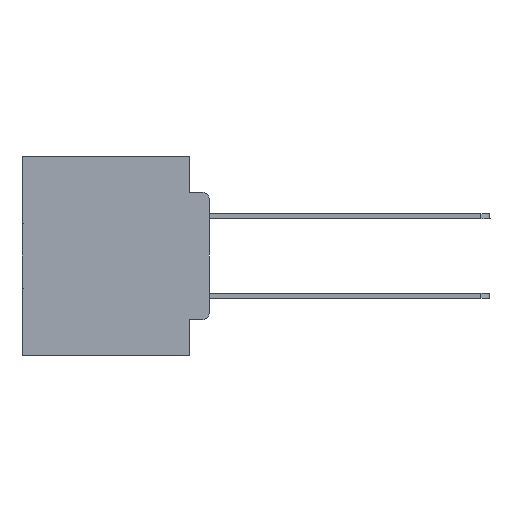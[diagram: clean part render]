
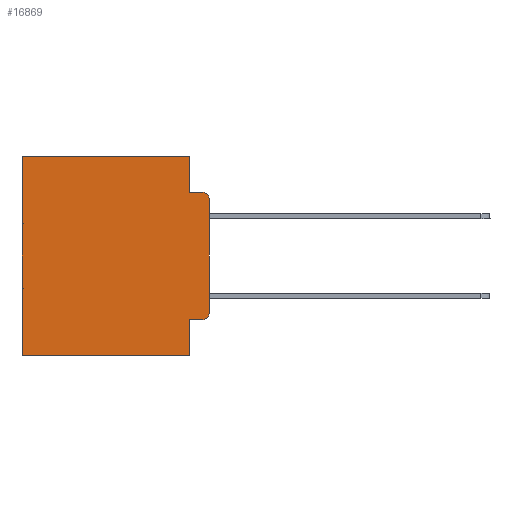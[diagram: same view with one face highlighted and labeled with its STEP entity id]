
A CAD part, left-side view. The second image highlights one B-rep face of the part: STEP entity #16869.
In plain terms, the highlighted planar face has unit normal (-1, 0, 0).
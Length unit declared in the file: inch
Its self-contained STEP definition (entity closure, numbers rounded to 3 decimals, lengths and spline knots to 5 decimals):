
#1502 = VERTEX_POINT ( 'NONE', #21563 ) ;
#1504 = VERTEX_POINT ( 'NONE', #26779 ) ;
#1955 = LINE ( 'NONE', #20442, #27430 ) ;
#2337 = EDGE_CURVE ( 'NONE', #17889, #27741, #2546, .T. ) ;
#2368 = DIRECTION ( 'NONE',  ( 1., 0., 0. ) ) ;
#2546 = LINE ( 'NONE', #7287, #12691 ) ;
#4616 = VERTEX_POINT ( 'NONE', #29684 ) ;
#5241 = VECTOR ( 'NONE', #23494, 39.37008 ) ;
#5605 = VECTOR ( 'NONE', #20570, 39.37008 ) ;
#6150 = AXIS2_PLACEMENT_3D ( 'NONE', #28214, #13589, #30662 ) ;
#6240 = CARTESIAN_POINT ( 'NONE',  ( 0.298, 0., 0. ) ) ;
#6424 = VERTEX_POINT ( 'NONE', #9900 ) ;
#6733 = CARTESIAN_POINT ( 'NONE',  ( 0.298, 0.473, 0. ) ) ;
#7261 = CARTESIAN_POINT ( 'NONE',  ( 0.298, 0., 0. ) ) ;
#7287 = CARTESIAN_POINT ( 'NONE',  ( 0.298, 0.051, -0.0885 ) ) ;
#7457 = DIRECTION ( 'NONE',  ( 0., -1., 0. ) ) ;
#7650 = LINE ( 'NONE', #17932, #9225 ) ;
#8582 = ORIENTED_EDGE ( 'NONE', *, *, #15921, .T. ) ;
#8660 = EDGE_CURVE ( 'NONE', #6424, #27741, #17504, .T. ) ;
#8824 = CARTESIAN_POINT ( 'NONE',  ( 0.298, 0.02, -0.3915 ) ) ;
#8850 = CARTESIAN_POINT ( 'NONE',  ( 0.298, 0.051, 0. ) ) ;
#9006 = EDGE_CURVE ( 'NONE', #14429, #17889, #31174, .T. ) ;
#9225 = VECTOR ( 'NONE', #25160, 39.37008 ) ;
#9534 = CARTESIAN_POINT ( 'NONE',  ( 0.298, 0., -0.5 ) ) ;
#9900 = CARTESIAN_POINT ( 'NONE',  ( 0.298, 0., -0.1085 ) ) ;
#10178 = ORIENTED_EDGE ( 'NONE', *, *, #29136, .T. ) ;
#10765 = DIRECTION ( 'NONE',  ( 0., 0., -1. ) ) ;
#11362 = DIRECTION ( 'NONE',  ( 0., 0., -1. ) ) ;
#11658 = VECTOR ( 'NONE', #10765, 39.37008 ) ;
#11864 = LINE ( 'NONE', #6240, #5241 ) ;
#12130 = DIRECTION ( 'NONE',  ( 0., -1., 0. ) ) ;
#12381 = CARTESIAN_POINT ( 'NONE',  ( 0.298, 0.473, -0.5 ) ) ;
#12691 = VECTOR ( 'NONE', #7457, 39.37008 ) ;
#12758 = EDGE_LOOP ( 'NONE', ( #29156, #12996, #13182, #12908, #10178, #31311, #23656, #28726, #15847, #8582 ) ) ;
#12908 = ORIENTED_EDGE ( 'NONE', *, *, #9006, .F. ) ;
#12996 = ORIENTED_EDGE ( 'NONE', *, *, #8660, .T. ) ;
#13182 = ORIENTED_EDGE ( 'NONE', *, *, #2337, .F. ) ;
#13232 = CIRCLE ( 'NONE', #23271, 0.02 ) ;
#13515 = LINE ( 'NONE', #26816, #20838 ) ;
#13589 = DIRECTION ( 'NONE',  ( -1., 0., 0. ) ) ;
#14429 = VERTEX_POINT ( 'NONE', #8850 ) ;
#15496 = EDGE_CURVE ( 'NONE', #21499, #31439, #24745, .T. ) ;
#15612 = DIRECTION ( 'NONE',  ( 0., 0., -1. ) ) ;
#15847 = ORIENTED_EDGE ( 'NONE', *, *, #20868, .T. ) ;
#15921 = EDGE_CURVE ( 'NONE', #4616, #1502, #13232, .T. ) ;
#16869 = ADVANCED_FACE ( 'NONE', ( #31117 ), #17280, .F. ) ;
#17280 = PLANE ( 'NONE',  #24705 ) ;
#17504 = CIRCLE ( 'NONE', #6150, 0.02 ) ;
#17889 = VERTEX_POINT ( 'NONE', #18810 ) ;
#17932 = CARTESIAN_POINT ( 'NONE',  ( 0.298, 0., 0. ) ) ;
#18111 = CARTESIAN_POINT ( 'NONE',  ( 0.298, 0.051, 0. ) ) ;
#18810 = CARTESIAN_POINT ( 'NONE',  ( 0.298, 0.051, -0.0885 ) ) ;
#19513 = DIRECTION ( 'NONE',  ( 0., 1., 0. ) ) ;
#19632 = CARTESIAN_POINT ( 'NONE',  ( 0.298, 0.02, -0.0885 ) ) ;
#19747 = DIRECTION ( 'NONE',  ( 0., 0., -1. ) ) ;
#20442 = CARTESIAN_POINT ( 'NONE',  ( 0.298, 0.473, 0. ) ) ;
#20570 = DIRECTION ( 'NONE',  ( 0., 0., -1. ) ) ;
#20838 = VECTOR ( 'NONE', #12130, 39.37008 ) ;
#20868 = EDGE_CURVE ( 'NONE', #1504, #4616, #13515, .T. ) ;
#21499 = VERTEX_POINT ( 'NONE', #21692 ) ;
#21563 = CARTESIAN_POINT ( 'NONE',  ( 0.298, 0., -0.3915 ) ) ;
#21692 = CARTESIAN_POINT ( 'NONE',  ( 0.298, 0.051, -0.5 ) ) ;
#22492 = EDGE_CURVE ( 'NONE', #1504, #21499, #24498, .T. ) ;
#23271 = AXIS2_PLACEMENT_3D ( 'NONE', #8824, #26044, #11362 ) ;
#23494 = DIRECTION ( 'NONE',  ( 0., 0., -1. ) ) ;
#23656 = ORIENTED_EDGE ( 'NONE', *, *, #15496, .F. ) ;
#24100 = EDGE_CURVE ( 'NONE', #29344, #31439, #1955, .T. ) ;
#24498 = LINE ( 'NONE', #18111, #5605 ) ;
#24705 = AXIS2_PLACEMENT_3D ( 'NONE', #7261, #2368, #19747 ) ;
#24745 = LINE ( 'NONE', #9534, #25503 ) ;
#25160 = DIRECTION ( 'NONE',  ( 0., 1., 0. ) ) ;
#25503 = VECTOR ( 'NONE', #19513, 39.37008 ) ;
#26044 = DIRECTION ( 'NONE',  ( -1., 0., 0. ) ) ;
#26779 = CARTESIAN_POINT ( 'NONE',  ( 0.298, 0.051, -0.4115 ) ) ;
#26816 = CARTESIAN_POINT ( 'NONE',  ( 0.298, 0.051, -0.4115 ) ) ;
#27430 = VECTOR ( 'NONE', #15612, 39.37008 ) ;
#27741 = VERTEX_POINT ( 'NONE', #19632 ) ;
#27910 = CARTESIAN_POINT ( 'NONE',  ( 0.298, 0.051, 0. ) ) ;
#28214 = CARTESIAN_POINT ( 'NONE',  ( 0.298, 0.02, -0.1085 ) ) ;
#28726 = ORIENTED_EDGE ( 'NONE', *, *, #22492, .F. ) ;
#29136 = EDGE_CURVE ( 'NONE', #14429, #29344, #7650, .T. ) ;
#29156 = ORIENTED_EDGE ( 'NONE', *, *, #30491, .F. ) ;
#29344 = VERTEX_POINT ( 'NONE', #6733 ) ;
#29684 = CARTESIAN_POINT ( 'NONE',  ( 0.298, 0.02, -0.4115 ) ) ;
#30491 = EDGE_CURVE ( 'NONE', #6424, #1502, #11864, .T. ) ;
#30662 = DIRECTION ( 'NONE',  ( 0., 0., -1. ) ) ;
#31117 = FACE_OUTER_BOUND ( 'NONE', #12758, .T. ) ;
#31174 = LINE ( 'NONE', #27910, #11658 ) ;
#31311 = ORIENTED_EDGE ( 'NONE', *, *, #24100, .T. ) ;
#31439 = VERTEX_POINT ( 'NONE', #12381 ) ;
